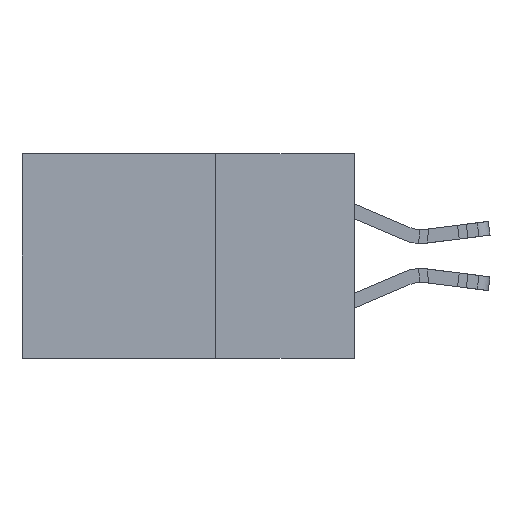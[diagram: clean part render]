
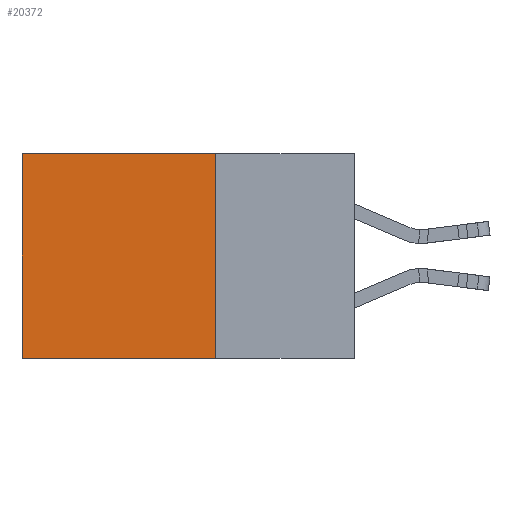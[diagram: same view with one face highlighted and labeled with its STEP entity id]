
A CAD part, left-side view. The second image highlights one B-rep face of the part: STEP entity #20372.
In plain terms, the highlighted planar face has unit normal (-1, 0, 0).
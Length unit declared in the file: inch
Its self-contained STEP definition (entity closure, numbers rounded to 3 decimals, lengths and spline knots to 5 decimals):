
#1980 = AXIS2_PLACEMENT_3D ( 'NONE', #19270, #12161, #7335 ) ;
#2381 = EDGE_CURVE ( 'NONE', #16172, #29260, #5273, .T. ) ;
#3617 = EDGE_CURVE ( 'NONE', #29260, #10215, #30177, .T. ) ;
#3829 = DIRECTION ( 'NONE',  ( 0., 1., 0. ) ) ;
#5273 = LINE ( 'NONE', #19174, #27699 ) ;
#6152 = ORIENTED_EDGE ( 'NONE', *, *, #3617, .F. ) ;
#6276 = DIRECTION ( 'NONE',  ( 0., 1., 0. ) ) ;
#6325 = EDGE_CURVE ( 'NONE', #8212, #10215, #13952, .T. ) ;
#7335 = DIRECTION ( 'NONE',  ( 0., 0., -1. ) ) ;
#8212 = VERTEX_POINT ( 'NONE', #18324 ) ;
#8892 = EDGE_LOOP ( 'NONE', ( #9193, #6152, #26273, #26153 ) ) ;
#9155 = CARTESIAN_POINT ( 'NONE',  ( 0.298, 0.6, 0. ) ) ;
#9193 = ORIENTED_EDGE ( 'NONE', *, *, #6325, .T. ) ;
#9485 = CARTESIAN_POINT ( 'NONE',  ( 0.298, 0.25, 0. ) ) ;
#9500 = CARTESIAN_POINT ( 'NONE',  ( 0.298, 0.6, -0.37 ) ) ;
#10215 = VERTEX_POINT ( 'NONE', #9500 ) ;
#10965 = CARTESIAN_POINT ( 'NONE',  ( 0.298, 0.25, -0.37 ) ) ;
#12095 = FACE_OUTER_BOUND ( 'NONE', #8892, .T. ) ;
#12161 = DIRECTION ( 'NONE',  ( 1., 0., 0. ) ) ;
#12232 = LINE ( 'NONE', #9485, #16362 ) ;
#12374 = PLANE ( 'NONE',  #1980 ) ;
#13277 = EDGE_CURVE ( 'NONE', #16172, #8212, #12232, .T. ) ;
#13952 = LINE ( 'NONE', #9155, #29632 ) ;
#14423 = DIRECTION ( 'NONE',  ( 0., 0., -1. ) ) ;
#16172 = VERTEX_POINT ( 'NONE', #24317 ) ;
#16362 = VECTOR ( 'NONE', #3829, 39.37008 ) ;
#16794 = DIRECTION ( 'NONE',  ( 0., 0., -1. ) ) ;
#18324 = CARTESIAN_POINT ( 'NONE',  ( 0.298, 0.6, 0. ) ) ;
#19174 = CARTESIAN_POINT ( 'NONE',  ( 0.298, 0.25, 0. ) ) ;
#19270 = CARTESIAN_POINT ( 'NONE',  ( 0.298, 0.25, 0. ) ) ;
#20372 = ADVANCED_FACE ( 'NONE', ( #12095 ), #12374, .F. ) ;
#20848 = VECTOR ( 'NONE', #6276, 39.37008 ) ;
#24317 = CARTESIAN_POINT ( 'NONE',  ( 0.298, 0.25, 0. ) ) ;
#26153 = ORIENTED_EDGE ( 'NONE', *, *, #13277, .T. ) ;
#26273 = ORIENTED_EDGE ( 'NONE', *, *, #2381, .F. ) ;
#27370 = CARTESIAN_POINT ( 'NONE',  ( 0.298, 0.25, -0.37 ) ) ;
#27699 = VECTOR ( 'NONE', #16794, 39.37008 ) ;
#29260 = VERTEX_POINT ( 'NONE', #27370 ) ;
#29632 = VECTOR ( 'NONE', #14423, 39.37008 ) ;
#30177 = LINE ( 'NONE', #10965, #20848 ) ;
